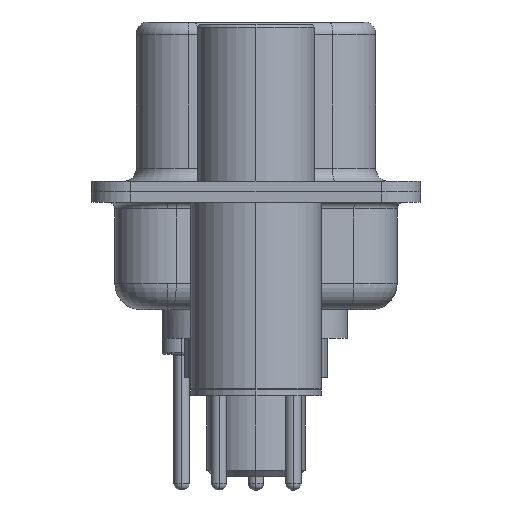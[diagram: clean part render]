
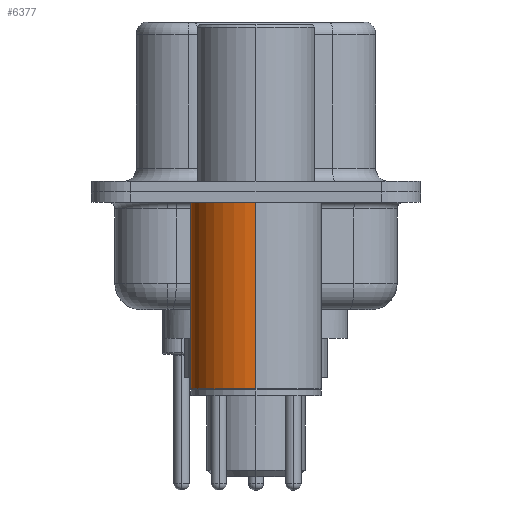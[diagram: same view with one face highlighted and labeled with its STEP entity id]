
A CAD part, left-side view. The second image highlights one B-rep face of the part: STEP entity #6377.
In plain terms, the highlighted cylindrical face has radius 2.5 mm (diameter 5 mm), a partial arc.
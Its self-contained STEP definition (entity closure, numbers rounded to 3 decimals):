
#85 = AXIS2_PLACEMENT_3D ( 'NONE', #10343, #5232, #15596 ) ;
#184 = VECTOR ( 'NONE', #19721, 1000. ) ;
#488 = VERTEX_POINT ( 'NONE', #19331 ) ;
#1313 = FACE_OUTER_BOUND ( 'NONE', #17370, .T. ) ;
#2346 = CARTESIAN_POINT ( 'NONE',  ( 0., 0., 0.581 ) ) ;
#3565 = ORIENTED_EDGE ( 'NONE', *, *, #5495, .T. ) ;
#3951 = CARTESIAN_POINT ( 'NONE',  ( 2.5, 0., 0.581 ) ) ;
#4500 = EDGE_CURVE ( 'NONE', #488, #20453, #12692, .T. ) ;
#4886 = AXIS2_PLACEMENT_3D ( 'NONE', #2346, #14532, #9326 ) ;
#5232 = DIRECTION ( 'NONE',  ( 0., 0., 1. ) ) ;
#5495 = EDGE_CURVE ( 'NONE', #488, #8594, #11397, .T. ) ;
#6377 = ADVANCED_FACE ( 'NONE', ( #1313 ), #19009, .T. ) ;
#7850 = CIRCLE ( 'NONE', #10289, 2.5 ) ;
#8594 = VERTEX_POINT ( 'NONE', #9340 ) ;
#9009 = DIRECTION ( 'NONE',  ( 0., 0., 1. ) ) ;
#9236 = CARTESIAN_POINT ( 'NONE',  ( 0., 0., -0.4 ) ) ;
#9326 = DIRECTION ( 'NONE',  ( 1., 0., 0. ) ) ;
#9340 = CARTESIAN_POINT ( 'NONE',  ( -2.5, 0., -7.525 ) ) ;
#10289 = AXIS2_PLACEMENT_3D ( 'NONE', #9236, #13205, #11520 ) ;
#10343 = CARTESIAN_POINT ( 'NONE',  ( 0., 0., -7.525 ) ) ;
#11069 = EDGE_CURVE ( 'NONE', #8594, #13805, #21780, .T. ) ;
#11397 = CIRCLE ( 'NONE', #85, 2.5 ) ;
#11520 = DIRECTION ( 'NONE',  ( 1., 0., 0. ) ) ;
#11751 = CARTESIAN_POINT ( 'NONE',  ( -2.5, 0., -0.4 ) ) ;
#11890 = EDGE_CURVE ( 'NONE', #20453, #13805, #7850, .T. ) ;
#12692 = LINE ( 'NONE', #3951, #184 ) ;
#13205 = DIRECTION ( 'NONE',  ( 0., 0., 1. ) ) ;
#13328 = ORIENTED_EDGE ( 'NONE', *, *, #11069, .T. ) ;
#13805 = VERTEX_POINT ( 'NONE', #11751 ) ;
#14532 = DIRECTION ( 'NONE',  ( 0., 0., 1. ) ) ;
#15570 = ORIENTED_EDGE ( 'NONE', *, *, #11890, .F. ) ;
#15596 = DIRECTION ( 'NONE',  ( 1., 0., 0. ) ) ;
#16948 = CARTESIAN_POINT ( 'NONE',  ( 2.5, 0., -0.4 ) ) ;
#17370 = EDGE_LOOP ( 'NONE', ( #3565, #13328, #15570, #21070 ) ) ;
#19009 = CYLINDRICAL_SURFACE ( 'NONE', #4886, 2.5 ) ;
#19331 = CARTESIAN_POINT ( 'NONE',  ( 2.5, 0., -7.525 ) ) ;
#19475 = CARTESIAN_POINT ( 'NONE',  ( -2.5, 0., 0.581 ) ) ;
#19721 = DIRECTION ( 'NONE',  ( 0., 0., 1. ) ) ;
#20453 = VERTEX_POINT ( 'NONE', #16948 ) ;
#21070 = ORIENTED_EDGE ( 'NONE', *, *, #4500, .F. ) ;
#21780 = LINE ( 'NONE', #19475, #22057 ) ;
#22057 = VECTOR ( 'NONE', #9009, 1000. ) ;
